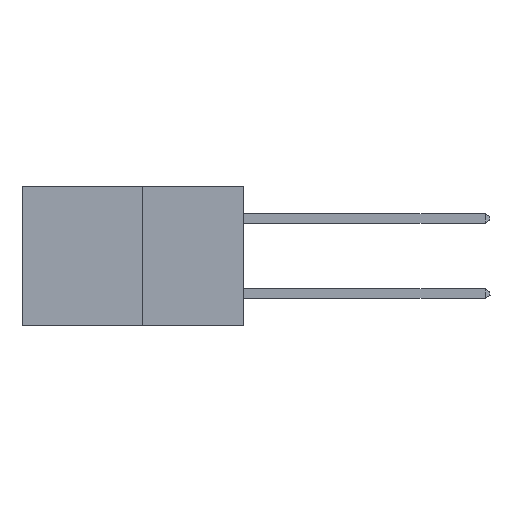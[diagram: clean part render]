
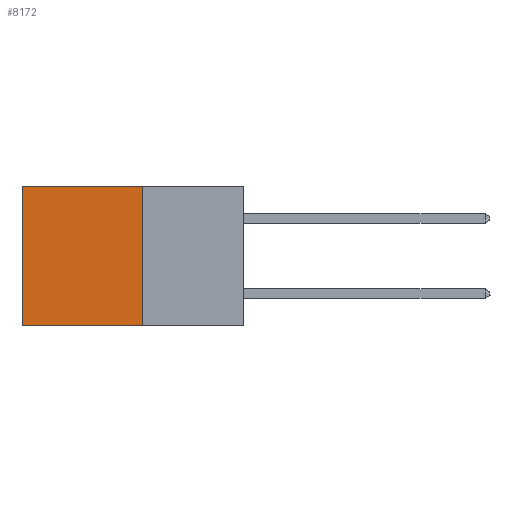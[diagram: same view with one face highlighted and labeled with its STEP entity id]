
A CAD part, left-side view. The second image highlights one B-rep face of the part: STEP entity #8172.
In plain terms, the highlighted planar face has unit normal (-1, 0, 0).
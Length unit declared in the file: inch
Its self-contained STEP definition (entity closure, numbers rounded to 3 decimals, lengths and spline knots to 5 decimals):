
#25 = LINE ( 'NONE', #10104, #11059 ) ;
#30 = EDGE_LOOP ( 'NONE', ( #7056, #6089, #10680, #10937 ) ) ;
#937 = CARTESIAN_POINT ( 'NONE',  ( 0.277, 0.59, 0. ) ) ;
#1512 = VECTOR ( 'NONE', #3528, 39.37008 ) ;
#2542 = DIRECTION ( 'NONE',  ( 0., 1., 0. ) ) ;
#2821 = VERTEX_POINT ( 'NONE', #937 ) ;
#3168 = FACE_OUTER_BOUND ( 'NONE', #30, .T. ) ;
#3251 = EDGE_CURVE ( 'NONE', #6604, #2821, #6406, .T. ) ;
#3334 = DIRECTION ( 'NONE',  ( 1., 0., 0. ) ) ;
#3528 = DIRECTION ( 'NONE',  ( 0., 0., -1. ) ) ;
#3653 = CARTESIAN_POINT ( 'NONE',  ( 0.277, 0.27, 0. ) ) ;
#4475 = CARTESIAN_POINT ( 'NONE',  ( 0.277, 0.59, -0.37 ) ) ;
#5786 = DIRECTION ( 'NONE',  ( 0., 0., -1. ) ) ;
#5819 = VECTOR ( 'NONE', #10502, 39.37008 ) ;
#5981 = EDGE_CURVE ( 'NONE', #6604, #9196, #25, .T. ) ;
#6089 = ORIENTED_EDGE ( 'NONE', *, *, #10997, .F. ) ;
#6208 = CARTESIAN_POINT ( 'NONE',  ( 0.277, 0.27, -0.37 ) ) ;
#6406 = LINE ( 'NONE', #3653, #10708 ) ;
#6604 = VERTEX_POINT ( 'NONE', #7430 ) ;
#7056 = ORIENTED_EDGE ( 'NONE', *, *, #9816, .T. ) ;
#7430 = CARTESIAN_POINT ( 'NONE',  ( 0.277, 0.27, 0. ) ) ;
#8172 = ADVANCED_FACE ( 'NONE', ( #3168 ), #8643, .F. ) ;
#8643 = PLANE ( 'NONE',  #11025 ) ;
#8669 = LINE ( 'NONE', #8812, #1512 ) ;
#8812 = CARTESIAN_POINT ( 'NONE',  ( 0.277, 0.59, -0.37 ) ) ;
#9196 = VERTEX_POINT ( 'NONE', #11420 ) ;
#9459 = CARTESIAN_POINT ( 'NONE',  ( 0.277, 0.27, -0.37 ) ) ;
#9496 = DIRECTION ( 'NONE',  ( 0., 0., -1. ) ) ;
#9816 = EDGE_CURVE ( 'NONE', #2821, #10472, #8669, .T. ) ;
#10104 = CARTESIAN_POINT ( 'NONE',  ( 0.277, 0.27, -0.37 ) ) ;
#10472 = VERTEX_POINT ( 'NONE', #4475 ) ;
#10502 = DIRECTION ( 'NONE',  ( 0., 1., 0. ) ) ;
#10680 = ORIENTED_EDGE ( 'NONE', *, *, #5981, .F. ) ;
#10696 = LINE ( 'NONE', #6208, #5819 ) ;
#10708 = VECTOR ( 'NONE', #2542, 39.37008 ) ;
#10937 = ORIENTED_EDGE ( 'NONE', *, *, #3251, .T. ) ;
#10997 = EDGE_CURVE ( 'NONE', #9196, #10472, #10696, .T. ) ;
#11025 = AXIS2_PLACEMENT_3D ( 'NONE', #9459, #3334, #9496 ) ;
#11059 = VECTOR ( 'NONE', #5786, 39.37008 ) ;
#11420 = CARTESIAN_POINT ( 'NONE',  ( 0.277, 0.27, -0.37 ) ) ;
